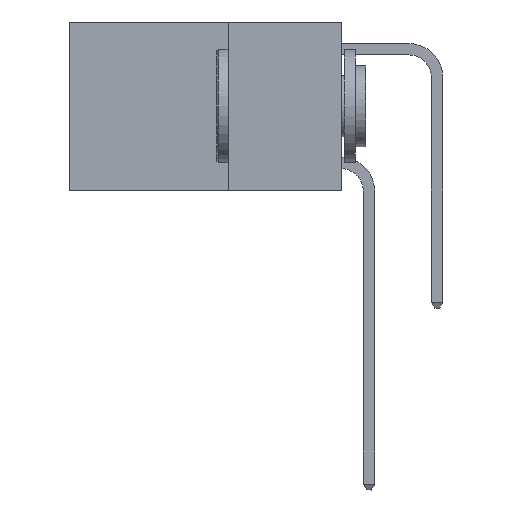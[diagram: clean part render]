
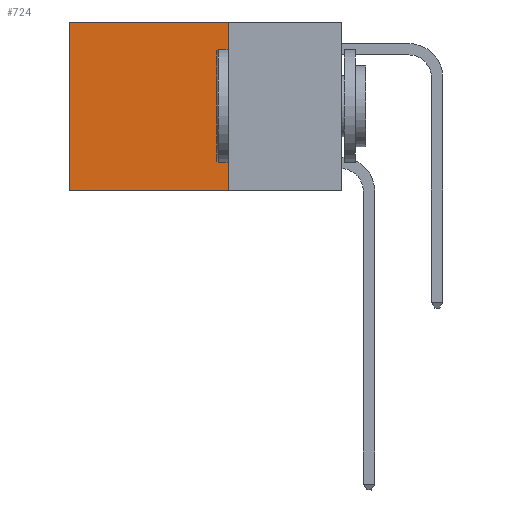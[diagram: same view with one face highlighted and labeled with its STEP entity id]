
A CAD part, left-side view. The second image highlights one B-rep face of the part: STEP entity #724.
In plain terms, the highlighted planar face has unit normal (-1, 0, 0).
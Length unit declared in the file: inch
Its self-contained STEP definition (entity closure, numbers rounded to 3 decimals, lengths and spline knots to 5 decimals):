
#254 = VERTEX_POINT ( 'NONE', #13306 ) ;
#391 = DIRECTION ( 'NONE',  ( 0., 0., -1. ) ) ;
#724 = ADVANCED_FACE ( 'NONE', ( #12766 ), #1157, .F. ) ;
#1047 = DIRECTION ( 'NONE',  ( 0., 0., -1. ) ) ;
#1059 = DIRECTION ( 'NONE',  ( 1., 0., 0. ) ) ;
#1105 = CARTESIAN_POINT ( 'NONE',  ( 0.2625, 0.25, 0. ) ) ;
#1157 = PLANE ( 'NONE',  #8176 ) ;
#1371 = LINE ( 'NONE', #13399, #9857 ) ;
#1849 = CARTESIAN_POINT ( 'NONE',  ( 0.2625, 0.25, 0. ) ) ;
#3296 = VECTOR ( 'NONE', #11463, 39.37008 ) ;
#3595 = ORIENTED_EDGE ( 'NONE', *, *, #7689, .F. ) ;
#5067 = VERTEX_POINT ( 'NONE', #6586 ) ;
#5988 = CARTESIAN_POINT ( 'NONE',  ( 0.2625, 0.25, -0.37 ) ) ;
#6472 = EDGE_CURVE ( 'NONE', #6962, #8905, #9177, .T. ) ;
#6586 = CARTESIAN_POINT ( 'NONE',  ( 0.2625, 0.25, -0.37 ) ) ;
#6962 = VERTEX_POINT ( 'NONE', #12466 ) ;
#7689 = EDGE_CURVE ( 'NONE', #254, #5067, #1371, .T. ) ;
#7729 = EDGE_CURVE ( 'NONE', #5067, #8905, #9138, .T. ) ;
#7748 = CARTESIAN_POINT ( 'NONE',  ( 0.2625, 0.6, 0. ) ) ;
#8176 = AXIS2_PLACEMENT_3D ( 'NONE', #1105, #1059, #1047 ) ;
#8700 = VECTOR ( 'NONE', #13681, 39.37008 ) ;
#8768 = CARTESIAN_POINT ( 'NONE',  ( 0.2625, 0.6, -0.37 ) ) ;
#8903 = DIRECTION ( 'NONE',  ( 0., 0., -1. ) ) ;
#8905 = VERTEX_POINT ( 'NONE', #8768 ) ;
#9096 = ORIENTED_EDGE ( 'NONE', *, *, #6472, .T. ) ;
#9133 = EDGE_CURVE ( 'NONE', #254, #6962, #11563, .T. ) ;
#9138 = LINE ( 'NONE', #5988, #3296 ) ;
#9177 = LINE ( 'NONE', #7748, #11349 ) ;
#9456 = ORIENTED_EDGE ( 'NONE', *, *, #9133, .T. ) ;
#9857 = VECTOR ( 'NONE', #391, 39.37008 ) ;
#11349 = VECTOR ( 'NONE', #8903, 39.37008 ) ;
#11463 = DIRECTION ( 'NONE',  ( 0., 1., 0. ) ) ;
#11563 = LINE ( 'NONE', #1849, #8700 ) ;
#11908 = ORIENTED_EDGE ( 'NONE', *, *, #7729, .F. ) ;
#12168 = EDGE_LOOP ( 'NONE', ( #9096, #11908, #3595, #9456 ) ) ;
#12466 = CARTESIAN_POINT ( 'NONE',  ( 0.2625, 0.6, 0. ) ) ;
#12766 = FACE_OUTER_BOUND ( 'NONE', #12168, .T. ) ;
#13306 = CARTESIAN_POINT ( 'NONE',  ( 0.2625, 0.25, 0. ) ) ;
#13399 = CARTESIAN_POINT ( 'NONE',  ( 0.2625, 0.25, 0. ) ) ;
#13681 = DIRECTION ( 'NONE',  ( 0., 1., 0. ) ) ;
